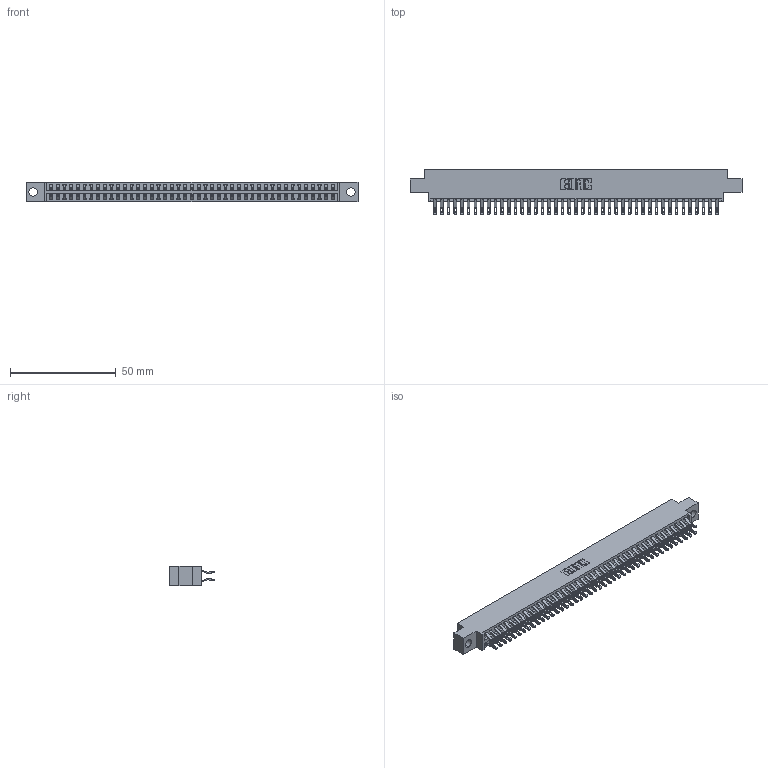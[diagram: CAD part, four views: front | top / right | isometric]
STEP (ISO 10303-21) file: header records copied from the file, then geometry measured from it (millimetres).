
FILE_DESCRIPTION (( 'STEP AP203' ), '1' );
FILE_NAME ('346-086-555-804.STEP', '2022-05-25T22:59:50', ( '' ), ( '' ), 'SwSTEP 2.0', 'SolidWorks 2020', '' );
FILE_SCHEMA (( 'CONFIG_CONTROL_DESIGN' ));
Length unit declared in the file: inch
Products named in the file (3): 346 Part_0.170 Offset - 0.156 Dia-TH; 345-292-001_555 Tail; 346-086-555-804
Assembly tree (87 placements, depth 2):
  346-086-555-804
    346 Part_0.170 Offset - 0.156 Dia-TH
    345-292-001_555 Tail  x86
Bounding box: 157.1 x 21.46 x 9.4 mm (x, y, z)
Volume: 15315.8 mm3; surface area: 21985 mm2
Topology: 87 solids, 87 shells, 5128 faces, 16115 edges, 10742 vertices
Faces by surface type: plane 2932, cylinder 2196
Entity records: 28805 total; most frequent: CARTESIAN_POINT 4788, ORIENTED_EDGE 4690, DIRECTION 4237, EDGE_CURVE 2345, VECTOR 2021, LINE 2021, VERTEX_POINT 1562, AXIS2_PLACEMENT_3D 1108
